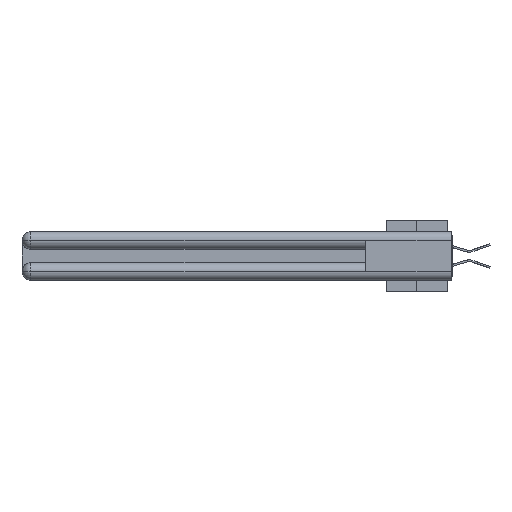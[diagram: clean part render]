
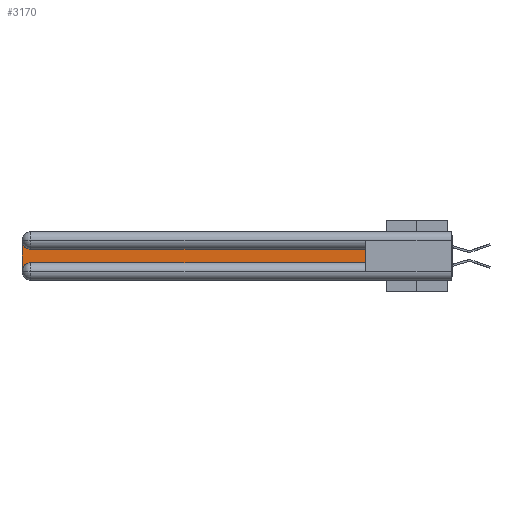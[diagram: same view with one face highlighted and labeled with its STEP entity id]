
A CAD part, left-side view. The second image highlights one B-rep face of the part: STEP entity #3170.
In plain terms, the highlighted planar face has unit normal (-1, 0, 0).
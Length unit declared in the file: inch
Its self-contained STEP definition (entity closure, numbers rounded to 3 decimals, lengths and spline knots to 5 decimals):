
#175 = LINE ( 'NONE', #32995, #33513 ) ;
#838 = VECTOR ( 'NONE', #36245, 39.37008 ) ;
#1507 = CARTESIAN_POINT ( 'NONE',  ( 0.075, 0.6, -0.1225 ) ) ;
#1634 = CARTESIAN_POINT ( 'NONE',  ( 0.075, 3., -0.2775 ) ) ;
#3170 = ADVANCED_FACE ( 'NONE', ( #14396 ), #33703, .F. ) ;
#4755 = CARTESIAN_POINT ( 'NONE',  ( 0.075, 0.6, -0.2175 ) ) ;
#5129 = EDGE_CURVE ( 'NONE', #25558, #12247, #21589, .T. ) ;
#8030 = DIRECTION ( 'NONE',  ( 0., 0., 1. ) ) ;
#8481 = VERTEX_POINT ( 'NONE', #40899 ) ;
#9909 = VECTOR ( 'NONE', #32871, 39.37008 ) ;
#10684 = DIRECTION ( 'NONE',  ( 1., 0., 0. ) ) ;
#10716 = EDGE_LOOP ( 'NONE', ( #22696, #41925, #39165, #25885, #14447, #14192 ) ) ;
#10959 = DIRECTION ( 'NONE',  ( 0., 0., -1. ) ) ;
#11024 = EDGE_CURVE ( 'NONE', #41857, #8481, #175, .T. ) ;
#12247 = VERTEX_POINT ( 'NONE', #13556 ) ;
#12347 = EDGE_CURVE ( 'NONE', #22823, #25558, #26211, .T. ) ;
#13556 = CARTESIAN_POINT ( 'NONE',  ( 0.075, 2.94, -0.2175 ) ) ;
#14192 = ORIENTED_EDGE ( 'NONE', *, *, #35936, .T. ) ;
#14261 = EDGE_CURVE ( 'NONE', #12247, #19358, #27147, .T. ) ;
#14396 = FACE_OUTER_BOUND ( 'NONE', #10716, .T. ) ;
#14447 = ORIENTED_EDGE ( 'NONE', *, *, #14261, .T. ) ;
#17310 = CARTESIAN_POINT ( 'NONE',  ( 0.075, 2.94, -0.0625 ) ) ;
#19358 = VERTEX_POINT ( 'NONE', #34875 ) ;
#19401 = AXIS2_PLACEMENT_3D ( 'NONE', #37082, #21029, #37338 ) ;
#19658 = CARTESIAN_POINT ( 'NONE',  ( 0.075, 3., -0.0625 ) ) ;
#19670 = CARTESIAN_POINT ( 'NONE',  ( 0.075, 2.94, -0.2775 ) ) ;
#21029 = DIRECTION ( 'NONE',  ( 1., 0., 0. ) ) ;
#21492 = VECTOR ( 'NONE', #8030, 39.37008 ) ;
#21589 = CIRCLE ( 'NONE', #34131, 0.06 ) ;
#22263 = EDGE_CURVE ( 'NONE', #8481, #22823, #28756, .T. ) ;
#22696 = ORIENTED_EDGE ( 'NONE', *, *, #11024, .T. ) ;
#22823 = VERTEX_POINT ( 'NONE', #19658 ) ;
#23043 = DIRECTION ( 'NONE',  ( 0., 1., 0. ) ) ;
#25558 = VERTEX_POINT ( 'NONE', #1634 ) ;
#25885 = ORIENTED_EDGE ( 'NONE', *, *, #5129, .T. ) ;
#25956 = DIRECTION ( 'NONE',  ( 1., 0., 0. ) ) ;
#26211 = LINE ( 'NONE', #39360, #838 ) ;
#26323 = CARTESIAN_POINT ( 'NONE',  ( 0.075, 0.6, -0.2175 ) ) ;
#26563 = LINE ( 'NONE', #4755, #21492 ) ;
#27147 = LINE ( 'NONE', #26323, #9909 ) ;
#27716 = AXIS2_PLACEMENT_3D ( 'NONE', #17310, #10684, #10959 ) ;
#28756 = CIRCLE ( 'NONE', #27716, 0.06 ) ;
#29102 = DIRECTION ( 'NONE',  ( 0., 0., -1. ) ) ;
#32871 = DIRECTION ( 'NONE',  ( 0., -1., 0. ) ) ;
#32995 = CARTESIAN_POINT ( 'NONE',  ( 0.075, 0.6, -0.1225 ) ) ;
#33513 = VECTOR ( 'NONE', #23043, 39.37008 ) ;
#33703 = PLANE ( 'NONE',  #19401 ) ;
#34131 = AXIS2_PLACEMENT_3D ( 'NONE', #19670, #25956, #29102 ) ;
#34875 = CARTESIAN_POINT ( 'NONE',  ( 0.075, 0.6, -0.2175 ) ) ;
#35936 = EDGE_CURVE ( 'NONE', #19358, #41857, #26563, .T. ) ;
#36245 = DIRECTION ( 'NONE',  ( 0., 0., -1. ) ) ;
#37082 = CARTESIAN_POINT ( 'NONE',  ( 0.075, 3., -0.1225 ) ) ;
#37338 = DIRECTION ( 'NONE',  ( 0., 0., -1. ) ) ;
#39165 = ORIENTED_EDGE ( 'NONE', *, *, #12347, .T. ) ;
#39360 = CARTESIAN_POINT ( 'NONE',  ( 0.075, 3., -0.2175 ) ) ;
#40899 = CARTESIAN_POINT ( 'NONE',  ( 0.075, 2.94, -0.1225 ) ) ;
#41857 = VERTEX_POINT ( 'NONE', #1507 ) ;
#41925 = ORIENTED_EDGE ( 'NONE', *, *, #22263, .T. ) ;
